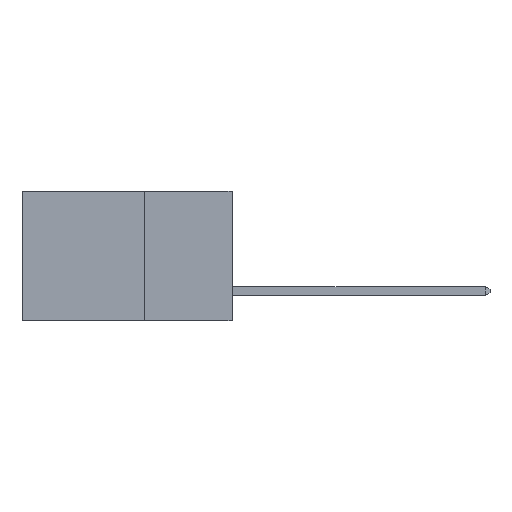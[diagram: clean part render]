
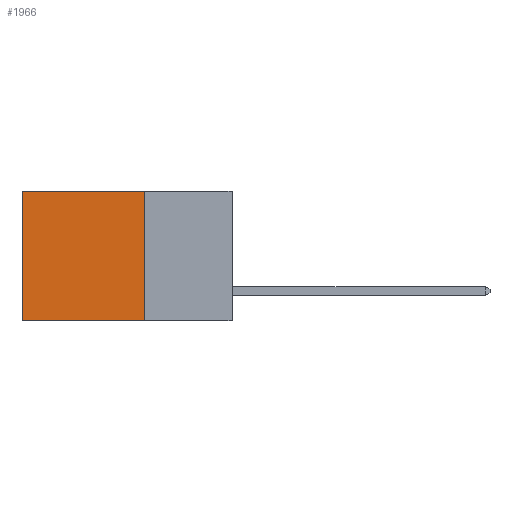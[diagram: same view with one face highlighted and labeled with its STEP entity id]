
A CAD part, left-side view. The second image highlights one B-rep face of the part: STEP entity #1966.
In plain terms, the highlighted planar face has unit normal (-1, 0, 0).
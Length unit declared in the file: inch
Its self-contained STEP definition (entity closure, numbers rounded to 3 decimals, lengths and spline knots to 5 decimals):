
#336 = LINE ( 'NONE', #32512, #13839 ) ;
#626 = DIRECTION ( 'NONE',  ( 0., 0., -1. ) ) ;
#1209 = CARTESIAN_POINT ( 'NONE',  ( 0.2875, 0.25, -0.37 ) ) ;
#1966 = ADVANCED_FACE ( 'NONE', ( #33159 ), #18561, .F. ) ;
#2096 = LINE ( 'NONE', #22863, #15602 ) ;
#3163 = CARTESIAN_POINT ( 'NONE',  ( 0.2875, 0.25, 0. ) ) ;
#3189 = LINE ( 'NONE', #30713, #4047 ) ;
#4047 = VECTOR ( 'NONE', #33326, 39.37008 ) ;
#4220 = VECTOR ( 'NONE', #11213, 39.37008 ) ;
#6901 = EDGE_CURVE ( 'NONE', #32496, #26289, #336, .T. ) ;
#7020 = VERTEX_POINT ( 'NONE', #1209 ) ;
#7698 = CARTESIAN_POINT ( 'NONE',  ( 0.2875, 0.25, 0. ) ) ;
#7949 = DIRECTION ( 'NONE',  ( 0., 0., -1. ) ) ;
#8476 = ORIENTED_EDGE ( 'NONE', *, *, #6901, .T. ) ;
#10491 = EDGE_LOOP ( 'NONE', ( #8476, #30519, #28175, #27966 ) ) ;
#11213 = DIRECTION ( 'NONE',  ( 0., 0., -1. ) ) ;
#12264 = LINE ( 'NONE', #3163, #4220 ) ;
#13311 = EDGE_CURVE ( 'NONE', #7020, #26289, #3189, .T. ) ;
#13839 = VECTOR ( 'NONE', #626, 39.37008 ) ;
#15602 = VECTOR ( 'NONE', #25541, 39.37008 ) ;
#16474 = EDGE_CURVE ( 'NONE', #20582, #7020, #12264, .T. ) ;
#16785 = AXIS2_PLACEMENT_3D ( 'NONE', #21214, #23857, #7949 ) ;
#18561 = PLANE ( 'NONE',  #16785 ) ;
#20231 = CARTESIAN_POINT ( 'NONE',  ( 0.2875, 0.6, -0.37 ) ) ;
#20582 = VERTEX_POINT ( 'NONE', #7698 ) ;
#21214 = CARTESIAN_POINT ( 'NONE',  ( 0.2875, 0.25, 0. ) ) ;
#22863 = CARTESIAN_POINT ( 'NONE',  ( 0.2875, 0.25, 0. ) ) ;
#23857 = DIRECTION ( 'NONE',  ( 1., 0., 0. ) ) ;
#25237 = CARTESIAN_POINT ( 'NONE',  ( 0.2875, 0.6, 0. ) ) ;
#25541 = DIRECTION ( 'NONE',  ( 0., 1., 0. ) ) ;
#26289 = VERTEX_POINT ( 'NONE', #20231 ) ;
#27381 = EDGE_CURVE ( 'NONE', #20582, #32496, #2096, .T. ) ;
#27966 = ORIENTED_EDGE ( 'NONE', *, *, #27381, .T. ) ;
#28175 = ORIENTED_EDGE ( 'NONE', *, *, #16474, .F. ) ;
#30519 = ORIENTED_EDGE ( 'NONE', *, *, #13311, .F. ) ;
#30713 = CARTESIAN_POINT ( 'NONE',  ( 0.2875, 0.25, -0.37 ) ) ;
#32496 = VERTEX_POINT ( 'NONE', #25237 ) ;
#32512 = CARTESIAN_POINT ( 'NONE',  ( 0.2875, 0.6, 0. ) ) ;
#33159 = FACE_OUTER_BOUND ( 'NONE', #10491, .T. ) ;
#33326 = DIRECTION ( 'NONE',  ( 0., 1., 0. ) ) ;
